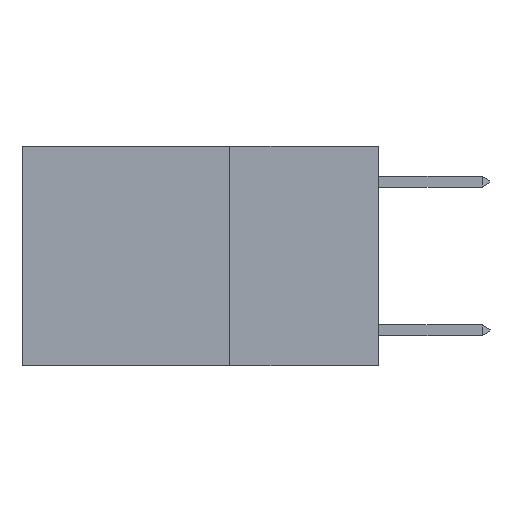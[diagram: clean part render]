
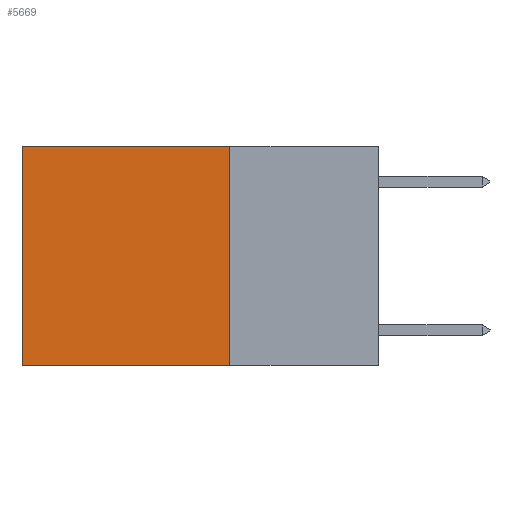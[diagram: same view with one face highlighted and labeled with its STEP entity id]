
A CAD part, left-side view. The second image highlights one B-rep face of the part: STEP entity #5669.
In plain terms, the highlighted planar face has unit normal (-1, 0, 0).
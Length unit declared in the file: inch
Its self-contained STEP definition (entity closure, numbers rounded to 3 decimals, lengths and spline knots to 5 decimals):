
#162 = CARTESIAN_POINT ( 'NONE',  ( 0.2625, 0.25, 0. ) ) ;
#239 = DIRECTION ( 'NONE',  ( 0., 1., 0. ) ) ;
#422 = DIRECTION ( 'NONE',  ( 0., 0., -1. ) ) ;
#951 = ORIENTED_EDGE ( 'NONE', *, *, #5397, .F. ) ;
#1179 = CARTESIAN_POINT ( 'NONE',  ( 0.2625, 0.6, 0. ) ) ;
#1229 = ORIENTED_EDGE ( 'NONE', *, *, #5209, .T. ) ;
#1543 = ORIENTED_EDGE ( 'NONE', *, *, #3944, .F. ) ;
#1982 = VECTOR ( 'NONE', #4885, 39.37008 ) ;
#2068 = EDGE_CURVE ( 'NONE', #7124, #4237, #4521, .T. ) ;
#2162 = CARTESIAN_POINT ( 'NONE',  ( 0.2625, 0.25, 0. ) ) ;
#2590 = CARTESIAN_POINT ( 'NONE',  ( 0.2625, 0.25, -0.37 ) ) ;
#3019 = DIRECTION ( 'NONE',  ( 0., 0., -1. ) ) ;
#3246 = CARTESIAN_POINT ( 'NONE',  ( 0.2625, 0.25, 0. ) ) ;
#3544 = ORIENTED_EDGE ( 'NONE', *, *, #2068, .T. ) ;
#3944 = EDGE_CURVE ( 'NONE', #7124, #5820, #4235, .T. ) ;
#4235 = LINE ( 'NONE', #3246, #1982 ) ;
#4237 = VERTEX_POINT ( 'NONE', #1179 ) ;
#4286 = FACE_OUTER_BOUND ( 'NONE', #8731, .T. ) ;
#4521 = LINE ( 'NONE', #162, #6897 ) ;
#4885 = DIRECTION ( 'NONE',  ( 0., 0., -1. ) ) ;
#5209 = EDGE_CURVE ( 'NONE', #4237, #5780, #6554, .T. ) ;
#5397 = EDGE_CURVE ( 'NONE', #5820, #5780, #6188, .T. ) ;
#5669 = ADVANCED_FACE ( 'NONE', ( #4286 ), #9194, .F. ) ;
#5780 = VERTEX_POINT ( 'NONE', #7885 ) ;
#5820 = VERTEX_POINT ( 'NONE', #7917 ) ;
#6188 = LINE ( 'NONE', #2590, #7699 ) ;
#6336 = CARTESIAN_POINT ( 'NONE',  ( 0.2625, 0.6, 0. ) ) ;
#6554 = LINE ( 'NONE', #6336, #10139 ) ;
#6633 = DIRECTION ( 'NONE',  ( 0., 1., 0. ) ) ;
#6897 = VECTOR ( 'NONE', #239, 39.37008 ) ;
#7124 = VERTEX_POINT ( 'NONE', #10253 ) ;
#7688 = AXIS2_PLACEMENT_3D ( 'NONE', #2162, #7743, #3019 ) ;
#7699 = VECTOR ( 'NONE', #6633, 39.37008 ) ;
#7743 = DIRECTION ( 'NONE',  ( 1., 0., 0. ) ) ;
#7885 = CARTESIAN_POINT ( 'NONE',  ( 0.2625, 0.6, -0.37 ) ) ;
#7917 = CARTESIAN_POINT ( 'NONE',  ( 0.2625, 0.25, -0.37 ) ) ;
#8731 = EDGE_LOOP ( 'NONE', ( #1229, #951, #1543, #3544 ) ) ;
#9194 = PLANE ( 'NONE',  #7688 ) ;
#10139 = VECTOR ( 'NONE', #422, 39.37008 ) ;
#10253 = CARTESIAN_POINT ( 'NONE',  ( 0.2625, 0.25, 0. ) ) ;
